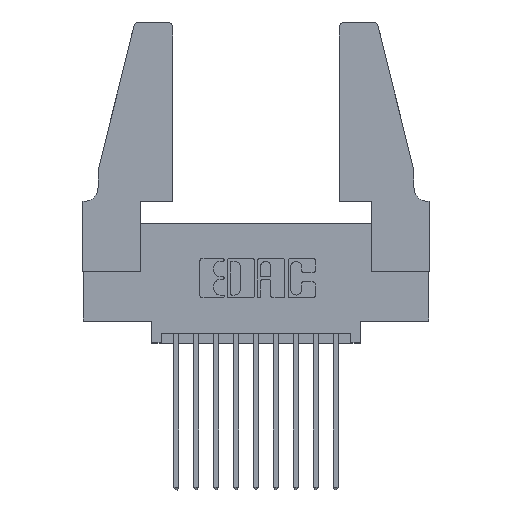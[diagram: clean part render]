
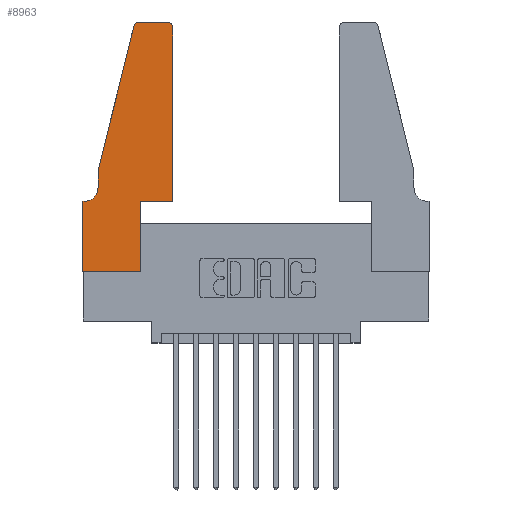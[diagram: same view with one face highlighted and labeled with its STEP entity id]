
A CAD part, top view. The second image highlights one B-rep face of the part: STEP entity #8963.
In plain terms, the highlighted planar face has unit normal (0, 0, 1).
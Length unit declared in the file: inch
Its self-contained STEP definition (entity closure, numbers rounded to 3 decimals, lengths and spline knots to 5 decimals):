
#117 = CARTESIAN_POINT ( 'NONE',  ( 0., 0., 0.37 ) ) ;
#402 = VERTEX_POINT ( 'NONE', #12866 ) ;
#541 = VECTOR ( 'NONE', #7648, 39.37008 ) ;
#704 = EDGE_CURVE ( 'NONE', #5750, #402, #11867, .T. ) ;
#797 = DIRECTION ( 'NONE',  ( 0., 0., 1. ) ) ;
#914 = DIRECTION ( 'NONE',  ( 0., 0., 1. ) ) ;
#1177 = AXIS2_PLACEMENT_3D ( 'NONE', #5155, #914, #8536 ) ;
#1499 = CARTESIAN_POINT ( 'NONE',  ( 0.25487, 1.22718, 0.37 ) ) ;
#1547 = LINE ( 'NONE', #9718, #541 ) ;
#1551 = ORIENTED_EDGE ( 'NONE', *, *, #11337, .T. ) ;
#1693 = ORIENTED_EDGE ( 'NONE', *, *, #7154, .T. ) ;
#2420 = ORIENTED_EDGE ( 'NONE', *, *, #8338, .T. ) ;
#2510 = ORIENTED_EDGE ( 'NONE', *, *, #4007, .T. ) ;
#2578 = AXIS2_PLACEMENT_3D ( 'NONE', #12394, #12529, #7181 ) ;
#2640 = VERTEX_POINT ( 'NONE', #13027 ) ;
#2652 = ORIENTED_EDGE ( 'NONE', *, *, #13671, .T. ) ;
#2861 = VECTOR ( 'NONE', #4342, 39.37008 ) ;
#2904 = DIRECTION ( 'NONE',  ( 1., 0., 0. ) ) ;
#3177 = CARTESIAN_POINT ( 'NONE',  ( 0.2865, 0.35, 0.37 ) ) ;
#3224 = VERTEX_POINT ( 'NONE', #10430 ) ;
#3327 = VERTEX_POINT ( 'NONE', #6443 ) ;
#3671 = LINE ( 'NONE', #6123, #5324 ) ;
#4007 = EDGE_CURVE ( 'NONE', #8509, #8466, #10133, .T. ) ;
#4050 = VERTEX_POINT ( 'NONE', #4093 ) ;
#4093 = CARTESIAN_POINT ( 'NONE',  ( 0., 0., 0.37 ) ) ;
#4151 = ORIENTED_EDGE ( 'NONE', *, *, #6408, .T. ) ;
#4286 = VECTOR ( 'NONE', #5378, 39.37008 ) ;
#4342 = DIRECTION ( 'NONE',  ( -1., 0., 0. ) ) ;
#4434 = EDGE_CURVE ( 'NONE', #402, #4050, #8805, .T. ) ;
#4485 = CARTESIAN_POINT ( 'NONE',  ( 0.4505, 0.35, 0.37 ) ) ;
#4560 = VECTOR ( 'NONE', #5606, 39.37008 ) ;
#4644 = CARTESIAN_POINT ( 'NONE',  ( 0.4505, 1.22, 0.37 ) ) ;
#4836 = AXIS2_PLACEMENT_3D ( 'NONE', #9754, #4941, #6068 ) ;
#4881 = FACE_OUTER_BOUND ( 'NONE', #13745, .T. ) ;
#4941 = DIRECTION ( 'NONE',  ( 0., 0., 1. ) ) ;
#5155 = CARTESIAN_POINT ( 'NONE',  ( 0., 0.35, 0.37 ) ) ;
#5324 = VECTOR ( 'NONE', #7209, 39.37008 ) ;
#5378 = DIRECTION ( 'NONE',  ( 0., 1., 0. ) ) ;
#5605 = VECTOR ( 'NONE', #11773, 39.37008 ) ;
#5606 = DIRECTION ( 'NONE',  ( 0., 1., 0. ) ) ;
#5750 = VERTEX_POINT ( 'NONE', #8254 ) ;
#5922 = CARTESIAN_POINT ( 'NONE',  ( 0.4205, 1.25, 0.37 ) ) ;
#6068 = DIRECTION ( 'NONE',  ( 1., 0., 0. ) ) ;
#6123 = CARTESIAN_POINT ( 'NONE',  ( 0., 0., 0.37 ) ) ;
#6161 = VERTEX_POINT ( 'NONE', #5922 ) ;
#6204 = CARTESIAN_POINT ( 'NONE',  ( 0.0755, 0.5, 0.37 ) ) ;
#6279 = VECTOR ( 'NONE', #13072, 39.37008 ) ;
#6408 = EDGE_CURVE ( 'NONE', #6161, #3327, #1547, .T. ) ;
#6434 = LINE ( 'NONE', #13120, #6279 ) ;
#6443 = CARTESIAN_POINT ( 'NONE',  ( 0.284, 1.25, 0.37 ) ) ;
#6524 = ORIENTED_EDGE ( 'NONE', *, *, #704, .T. ) ;
#6862 = ORIENTED_EDGE ( 'NONE', *, *, #11309, .T. ) ;
#7154 = EDGE_CURVE ( 'NONE', #3327, #12331, #11930, .T. ) ;
#7181 = DIRECTION ( 'NONE',  ( -1., 0., 0. ) ) ;
#7209 = DIRECTION ( 'NONE',  ( 1., 0., 0. ) ) ;
#7385 = DIRECTION ( 'NONE',  ( 1., 0., 0. ) ) ;
#7434 = LINE ( 'NONE', #4485, #4560 ) ;
#7437 = CARTESIAN_POINT ( 'NONE',  ( 0.4505, 0.35, 0.37 ) ) ;
#7648 = DIRECTION ( 'NONE',  ( -1., 0., 0. ) ) ;
#7982 = VECTOR ( 'NONE', #7385, 39.37008 ) ;
#8169 = LINE ( 'NONE', #3177, #4286 ) ;
#8254 = CARTESIAN_POINT ( 'NONE',  ( 0.0055, 0.35, 0.37 ) ) ;
#8338 = EDGE_CURVE ( 'NONE', #8466, #13518, #7434, .T. ) ;
#8466 = VERTEX_POINT ( 'NONE', #11245 ) ;
#8479 = DIRECTION ( 'NONE',  ( -0.239, -0.971, 0. ) ) ;
#8509 = VERTEX_POINT ( 'NONE', #13831 ) ;
#8536 = DIRECTION ( 'NONE',  ( 1., 0., 0. ) ) ;
#8577 = ORIENTED_EDGE ( 'NONE', *, *, #9335, .T. ) ;
#8805 = LINE ( 'NONE', #117, #5605 ) ;
#8918 = VECTOR ( 'NONE', #8479, 39.37008 ) ;
#8963 = ADVANCED_FACE ( 'NONE', ( #4881 ), #12812, .T. ) ;
#9335 = EDGE_CURVE ( 'NONE', #13518, #6161, #11555, .T. ) ;
#9718 = CARTESIAN_POINT ( 'NONE',  ( 0.2605, 1.25, 0.37 ) ) ;
#9754 = CARTESIAN_POINT ( 'NONE',  ( 0.284, 1.22, 0.37 ) ) ;
#9887 = VERTEX_POINT ( 'NONE', #10696 ) ;
#10133 = LINE ( 'NONE', #7437, #7982 ) ;
#10430 = CARTESIAN_POINT ( 'NONE',  ( 0.0755, 0.42, 0.37 ) ) ;
#10696 = CARTESIAN_POINT ( 'NONE',  ( 0.2865, 0., 0.37 ) ) ;
#11103 = AXIS2_PLACEMENT_3D ( 'NONE', #12375, #797, #2904 ) ;
#11245 = CARTESIAN_POINT ( 'NONE',  ( 0.4505, 0.35, 0.37 ) ) ;
#11293 = ORIENTED_EDGE ( 'NONE', *, *, #4434, .T. ) ;
#11309 = EDGE_CURVE ( 'NONE', #4050, #9887, #3671, .T. ) ;
#11337 = EDGE_CURVE ( 'NONE', #9887, #8509, #8169, .T. ) ;
#11437 = ORIENTED_EDGE ( 'NONE', *, *, #13235, .T. ) ;
#11555 = CIRCLE ( 'NONE', #11103, 0.03 ) ;
#11577 = LINE ( 'NONE', #6204, #8918 ) ;
#11773 = DIRECTION ( 'NONE',  ( 0., -1., 0. ) ) ;
#11867 = LINE ( 'NONE', #12769, #2861 ) ;
#11930 = CIRCLE ( 'NONE', #4836, 0.03 ) ;
#12331 = VERTEX_POINT ( 'NONE', #1499 ) ;
#12375 = CARTESIAN_POINT ( 'NONE',  ( 0.4205, 1.22, 0.37 ) ) ;
#12394 = CARTESIAN_POINT ( 'NONE',  ( 0.0055, 0.42, 0.37 ) ) ;
#12529 = DIRECTION ( 'NONE',  ( 0., 0., -1. ) ) ;
#12734 = CIRCLE ( 'NONE', #2578, 0.07 ) ;
#12769 = CARTESIAN_POINT ( 'NONE',  ( 0.0755, 0.35, 0.37 ) ) ;
#12812 = PLANE ( 'NONE',  #1177 ) ;
#12866 = CARTESIAN_POINT ( 'NONE',  ( 0., 0.35, 0.37 ) ) ;
#12918 = EDGE_CURVE ( 'NONE', #2640, #3224, #6434, .T. ) ;
#13027 = CARTESIAN_POINT ( 'NONE',  ( 0.0755, 0.5, 0.37 ) ) ;
#13072 = DIRECTION ( 'NONE',  ( 0., -1., 0. ) ) ;
#13120 = CARTESIAN_POINT ( 'NONE',  ( 0.0755, 0.5, 0.37 ) ) ;
#13235 = EDGE_CURVE ( 'NONE', #12331, #2640, #11577, .T. ) ;
#13300 = ORIENTED_EDGE ( 'NONE', *, *, #12918, .T. ) ;
#13518 = VERTEX_POINT ( 'NONE', #4644 ) ;
#13671 = EDGE_CURVE ( 'NONE', #3224, #5750, #12734, .T. ) ;
#13745 = EDGE_LOOP ( 'NONE', ( #4151, #1693, #11437, #13300, #2652, #6524, #11293, #6862, #1551, #2510, #2420, #8577 ) ) ;
#13831 = CARTESIAN_POINT ( 'NONE',  ( 0.2865, 0.35, 0.37 ) ) ;
